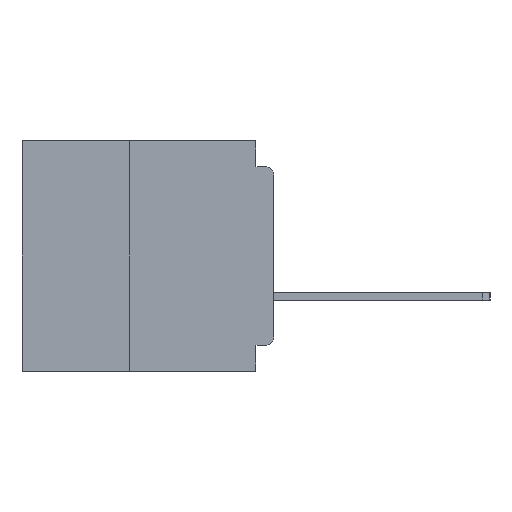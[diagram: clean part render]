
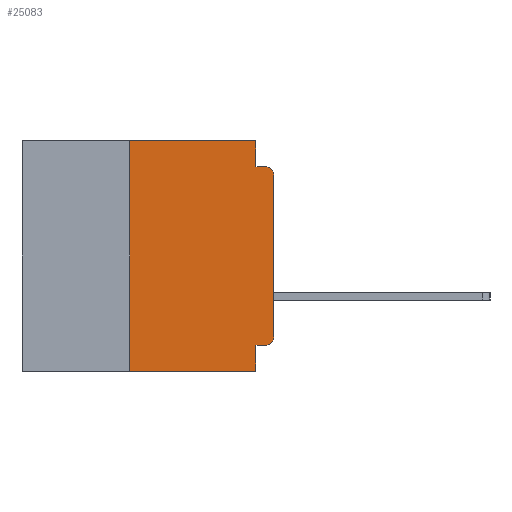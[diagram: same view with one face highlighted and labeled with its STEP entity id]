
A CAD part, left-side view. The second image highlights one B-rep face of the part: STEP entity #25083.
In plain terms, the highlighted planar face has unit normal (-1, 0, 0).
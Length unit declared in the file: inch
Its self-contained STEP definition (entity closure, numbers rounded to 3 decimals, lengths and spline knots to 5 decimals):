
#94 = CARTESIAN_POINT ( 'NONE',  ( 0., 0., 0. ) ) ;
#494 = DIRECTION ( 'NONE',  ( 0., 0., -1. ) ) ;
#783 = AXIS2_PLACEMENT_3D ( 'NONE', #31853, #2513, #36748 ) ;
#1208 = VERTEX_POINT ( 'NONE', #26742 ) ;
#2050 = DIRECTION ( 'NONE',  ( 1., 0., 0. ) ) ;
#2175 = VERTEX_POINT ( 'NONE', #29660 ) ;
#2513 = DIRECTION ( 'NONE',  ( -1., 0., 0. ) ) ;
#2654 = LINE ( 'NONE', #39286, #4185 ) ;
#4185 = VECTOR ( 'NONE', #44186, 39.37008 ) ;
#5816 = VERTEX_POINT ( 'NONE', #34262 ) ;
#6593 = ORIENTED_EDGE ( 'NONE', *, *, #47370, .T. ) ;
#7167 = CIRCLE ( 'NONE', #46762, 0.015 ) ;
#7225 = CARTESIAN_POINT ( 'NONE',  ( 0., 0.437, -0.4 ) ) ;
#7696 = CARTESIAN_POINT ( 'NONE',  ( 0., 0.25, -0.4 ) ) ;
#7891 = AXIS2_PLACEMENT_3D ( 'NONE', #31405, #2050, #36303 ) ;
#8974 = ORIENTED_EDGE ( 'NONE', *, *, #51684, .F. ) ;
#10443 = LINE ( 'NONE', #94, #36449 ) ;
#11414 = LINE ( 'NONE', #26006, #50402 ) ;
#11587 = DIRECTION ( 'NONE',  ( 0., -1., 0. ) ) ;
#11630 = ORIENTED_EDGE ( 'NONE', *, *, #26152, .F. ) ;
#11648 = ORIENTED_EDGE ( 'NONE', *, *, #36941, .T. ) ;
#11883 = ORIENTED_EDGE ( 'NONE', *, *, #28809, .T. ) ;
#12282 = CIRCLE ( 'NONE', #783, 0.015 ) ;
#13214 = ORIENTED_EDGE ( 'NONE', *, *, #21170, .F. ) ;
#14642 = VECTOR ( 'NONE', #41956, 39.37008 ) ;
#15346 = ORIENTED_EDGE ( 'NONE', *, *, #53798, .F. ) ;
#15648 = LINE ( 'NONE', #36681, #40137 ) ;
#16636 = PLANE ( 'NONE',  #7891 ) ;
#18488 = ORIENTED_EDGE ( 'NONE', *, *, #23537, .F. ) ;
#21170 = EDGE_CURVE ( 'NONE', #5816, #2175, #11414, .T. ) ;
#23537 = EDGE_CURVE ( 'NONE', #33090, #5816, #2654, .T. ) ;
#25083 = ADVANCED_FACE ( 'NONE', ( #27079 ), #16636, .F. ) ;
#25543 = ORIENTED_EDGE ( 'NONE', *, *, #62798, .T. ) ;
#26006 = CARTESIAN_POINT ( 'NONE',  ( 0., 0., -0.045 ) ) ;
#26128 = LINE ( 'NONE', #7696, #14642 ) ;
#26152 = EDGE_CURVE ( 'NONE', #43346, #1208, #26128, .T. ) ;
#26742 = CARTESIAN_POINT ( 'NONE',  ( 0., 0.25, 0. ) ) ;
#27079 = FACE_OUTER_BOUND ( 'NONE', #48415, .T. ) ;
#28809 = EDGE_CURVE ( 'NONE', #43346, #49501, #54948, .T. ) ;
#29513 = VERTEX_POINT ( 'NONE', #62112 ) ;
#29660 = CARTESIAN_POINT ( 'NONE',  ( 0., 0.015, -0.045 ) ) ;
#29877 = DIRECTION ( 'NONE',  ( -1., 0., 0. ) ) ;
#30224 = CARTESIAN_POINT ( 'NONE',  ( 0., 0.031, 0. ) ) ;
#31216 = CARTESIAN_POINT ( 'NONE',  ( 0., 0.25, -0.4 ) ) ;
#31405 = CARTESIAN_POINT ( 'NONE',  ( 0., 0.437, 0. ) ) ;
#31853 = CARTESIAN_POINT ( 'NONE',  ( 0., 0.015, -0.34 ) ) ;
#32398 = CARTESIAN_POINT ( 'NONE',  ( 0., 0.031, -0.4 ) ) ;
#32689 = ORIENTED_EDGE ( 'NONE', *, *, #53240, .F. ) ;
#33090 = VERTEX_POINT ( 'NONE', #30224 ) ;
#34262 = CARTESIAN_POINT ( 'NONE',  ( 0., 0.031, -0.045 ) ) ;
#35999 = CARTESIAN_POINT ( 'NONE',  ( 0., 0.437, 0. ) ) ;
#36303 = DIRECTION ( 'NONE',  ( 0., 0., -1. ) ) ;
#36449 = VECTOR ( 'NONE', #39301, 39.37008 ) ;
#36681 = CARTESIAN_POINT ( 'NONE',  ( 0., 0., -0.355 ) ) ;
#36748 = DIRECTION ( 'NONE',  ( 0., 0., -1. ) ) ;
#36941 = EDGE_CURVE ( 'NONE', #29513, #42032, #10443, .T. ) ;
#39286 = CARTESIAN_POINT ( 'NONE',  ( 0., 0.031, 0. ) ) ;
#39301 = DIRECTION ( 'NONE',  ( 0., 0., 1. ) ) ;
#40110 = CARTESIAN_POINT ( 'NONE',  ( 0., 0., -0.06 ) ) ;
#40137 = VECTOR ( 'NONE', #41598, 39.37008 ) ;
#41471 = DIRECTION ( 'NONE',  ( 0., -1., 0. ) ) ;
#41598 = DIRECTION ( 'NONE',  ( 0., 1., 0. ) ) ;
#41956 = DIRECTION ( 'NONE',  ( 0., 0., 1. ) ) ;
#42032 = VERTEX_POINT ( 'NONE', #40110 ) ;
#43346 = VERTEX_POINT ( 'NONE', #31216 ) ;
#44186 = DIRECTION ( 'NONE',  ( 0., 0., -1. ) ) ;
#44741 = VECTOR ( 'NONE', #59796, 39.37008 ) ;
#46762 = AXIS2_PLACEMENT_3D ( 'NONE', #58937, #29877, #494 ) ;
#47370 = EDGE_CURVE ( 'NONE', #57709, #29513, #12282, .T. ) ;
#48095 = VERTEX_POINT ( 'NONE', #59722 ) ;
#48415 = EDGE_LOOP ( 'NONE', ( #11648, #25543, #13214, #18488, #15346, #11630, #11883, #32689, #8974, #6593 ) ) ;
#48461 = VECTOR ( 'NONE', #11587, 39.37008 ) ;
#49501 = VERTEX_POINT ( 'NONE', #32398 ) ;
#50402 = VECTOR ( 'NONE', #55143, 39.37008 ) ;
#51684 = EDGE_CURVE ( 'NONE', #57709, #48095, #15648, .T. ) ;
#51959 = CARTESIAN_POINT ( 'NONE',  ( 0., 0.015, -0.355 ) ) ;
#53240 = EDGE_CURVE ( 'NONE', #48095, #49501, #57553, .T. ) ;
#53798 = EDGE_CURVE ( 'NONE', #1208, #33090, #61272, .T. ) ;
#54948 = LINE ( 'NONE', #7225, #57934 ) ;
#54957 = CARTESIAN_POINT ( 'NONE',  ( 0., 0.031, -0.4 ) ) ;
#55143 = DIRECTION ( 'NONE',  ( 0., -1., 0. ) ) ;
#57553 = LINE ( 'NONE', #54957, #44741 ) ;
#57709 = VERTEX_POINT ( 'NONE', #51959 ) ;
#57934 = VECTOR ( 'NONE', #41471, 39.37008 ) ;
#58937 = CARTESIAN_POINT ( 'NONE',  ( 0., 0.015, -0.06 ) ) ;
#59722 = CARTESIAN_POINT ( 'NONE',  ( 0., 0.031, -0.355 ) ) ;
#59796 = DIRECTION ( 'NONE',  ( 0., 0., -1. ) ) ;
#61272 = LINE ( 'NONE', #35999, #48461 ) ;
#62112 = CARTESIAN_POINT ( 'NONE',  ( 0., 0., -0.34 ) ) ;
#62798 = EDGE_CURVE ( 'NONE', #42032, #2175, #7167, .T. ) ;
